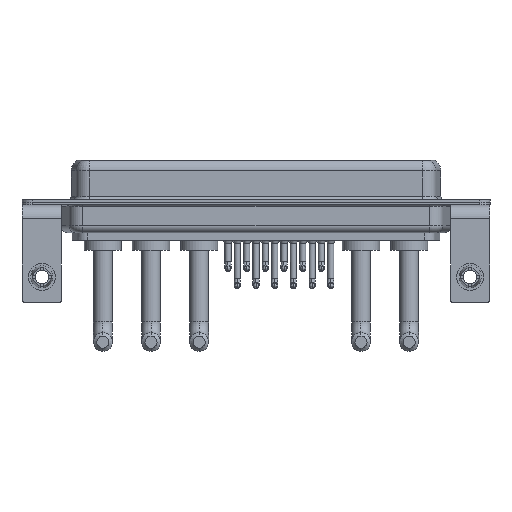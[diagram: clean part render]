
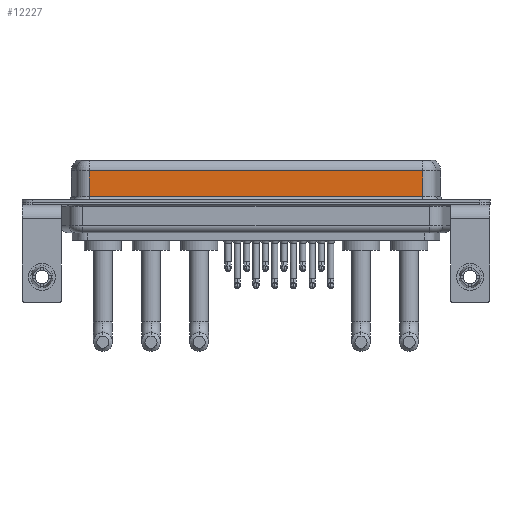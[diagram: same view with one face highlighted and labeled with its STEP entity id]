
A CAD part, front view. The second image highlights one B-rep face of the part: STEP entity #12227.
In plain terms, the highlighted planar face has unit normal (0, -1, 0).
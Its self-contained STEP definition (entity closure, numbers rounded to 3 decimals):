
#923 = ORIENTED_EDGE ( 'NONE', *, *, #10711, .T. ) ;
#1355 = EDGE_CURVE ( 'NONE', #1372, #9207, #1566, .T. ) ;
#1372 = VERTEX_POINT ( 'NONE', #5225 ) ;
#1566 = LINE ( 'NONE', #7068, #18922 ) ;
#1601 = CARTESIAN_POINT ( 'NONE',  ( 7.038, -3.95, 0.9 ) ) ;
#1670 = CARTESIAN_POINT ( 'NONE',  ( 56.462, -3.95, 6.4 ) ) ;
#1870 = VECTOR ( 'NONE', #21142, 1000. ) ;
#2480 = ORIENTED_EDGE ( 'NONE', *, *, #13083, .F. ) ;
#2723 = CARTESIAN_POINT ( 'NONE',  ( 56.462, -3.95, 4.65 ) ) ;
#2747 = EDGE_CURVE ( 'NONE', #9207, #13460, #5825, .T. ) ;
#2990 = ORIENTED_EDGE ( 'NONE', *, *, #2747, .T. ) ;
#3436 = CARTESIAN_POINT ( 'NONE',  ( 56.462, -3.95, 6.4 ) ) ;
#4756 = VECTOR ( 'NONE', #18066, 1000. ) ;
#5204 = VERTEX_POINT ( 'NONE', #2723 ) ;
#5225 = CARTESIAN_POINT ( 'NONE',  ( 7.038, -3.95, 4.65 ) ) ;
#5825 = LINE ( 'NONE', #11068, #4756 ) ;
#7068 = CARTESIAN_POINT ( 'NONE',  ( 7.038, -3.95, 6.4 ) ) ;
#7180 = DIRECTION ( 'NONE',  ( 0., 0., -1. ) ) ;
#7270 = PLANE ( 'NONE',  #12470 ) ;
#7719 = DIRECTION ( 'NONE',  ( 0., 1., 0. ) ) ;
#7887 = CARTESIAN_POINT ( 'NONE',  ( 56.462, -3.95, 0.9 ) ) ;
#8091 = ORIENTED_EDGE ( 'NONE', *, *, #1355, .T. ) ;
#8126 = VECTOR ( 'NONE', #15904, 1000. ) ;
#9207 = VERTEX_POINT ( 'NONE', #1601 ) ;
#10500 = LINE ( 'NONE', #19090, #1870 ) ;
#10711 = EDGE_CURVE ( 'NONE', #5204, #1372, #10500, .T. ) ;
#11068 = CARTESIAN_POINT ( 'NONE',  ( 56.462, -3.95, 0.9 ) ) ;
#12005 = LINE ( 'NONE', #3436, #8126 ) ;
#12227 = ADVANCED_FACE ( 'NONE', ( #21091 ), #7270, .F. ) ;
#12470 = AXIS2_PLACEMENT_3D ( 'NONE', #1670, #7719, #14699 ) ;
#13083 = EDGE_CURVE ( 'NONE', #5204, #13460, #12005, .T. ) ;
#13460 = VERTEX_POINT ( 'NONE', #7887 ) ;
#14699 = DIRECTION ( 'NONE',  ( 0., 0., 1. ) ) ;
#15904 = DIRECTION ( 'NONE',  ( 0., 0., -1. ) ) ;
#16050 = EDGE_LOOP ( 'NONE', ( #2480, #923, #8091, #2990 ) ) ;
#18066 = DIRECTION ( 'NONE',  ( 1., 0., 0. ) ) ;
#18922 = VECTOR ( 'NONE', #7180, 1000. ) ;
#19090 = CARTESIAN_POINT ( 'NONE',  ( 56.462, -3.95, 4.65 ) ) ;
#21091 = FACE_OUTER_BOUND ( 'NONE', #16050, .T. ) ;
#21142 = DIRECTION ( 'NONE',  ( -1., 0., 0. ) ) ;
